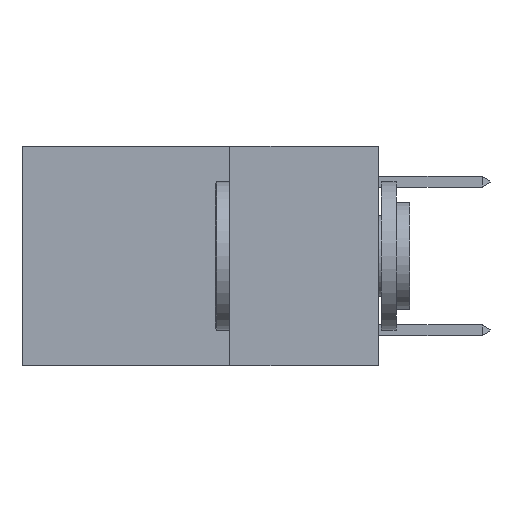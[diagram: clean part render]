
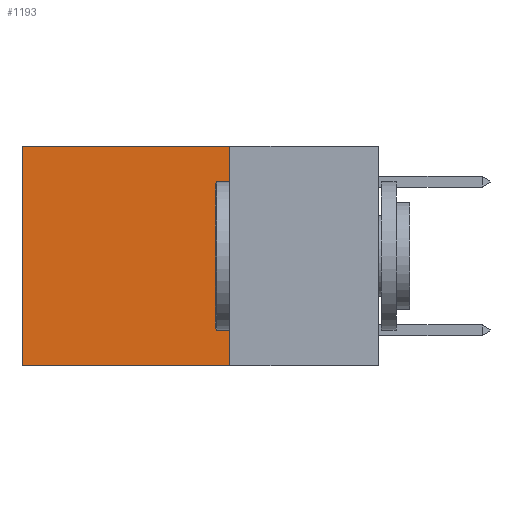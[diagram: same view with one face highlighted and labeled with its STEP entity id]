
A CAD part, left-side view. The second image highlights one B-rep face of the part: STEP entity #1193.
In plain terms, the highlighted planar face has unit normal (-1, 0, 0).
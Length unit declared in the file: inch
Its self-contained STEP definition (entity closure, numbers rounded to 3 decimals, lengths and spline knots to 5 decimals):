
#996 = ORIENTED_EDGE ( 'NONE', *, *, #20381, .F. ) ;
#1029 = LINE ( 'NONE', #21350, #8404 ) ;
#1193 = ADVANCED_FACE ( 'NONE', ( #12612 ), #3220, .F. ) ;
#1572 = CARTESIAN_POINT ( 'NONE',  ( 0.2625, 0.6, 0. ) ) ;
#2079 = DIRECTION ( 'NONE',  ( 0., 1., 0. ) ) ;
#3168 = EDGE_CURVE ( 'NONE', #18322, #13015, #1029, .T. ) ;
#3220 = PLANE ( 'NONE',  #7513 ) ;
#3239 = DIRECTION ( 'NONE',  ( 0., 0., -1. ) ) ;
#3312 = CARTESIAN_POINT ( 'NONE',  ( 0.2625, 0.25, 0. ) ) ;
#4882 = VERTEX_POINT ( 'NONE', #9072 ) ;
#4938 = DIRECTION ( 'NONE',  ( 0., 0., -1. ) ) ;
#7513 = AXIS2_PLACEMENT_3D ( 'NONE', #18361, #14005, #21629 ) ;
#8404 = VECTOR ( 'NONE', #16106, 39.37008 ) ;
#8825 = EDGE_CURVE ( 'NONE', #13015, #11141, #14647, .T. ) ;
#9072 = CARTESIAN_POINT ( 'NONE',  ( 0.2625, 0.25, -0.37 ) ) ;
#9476 = LINE ( 'NONE', #16934, #18950 ) ;
#9788 = EDGE_CURVE ( 'NONE', #18322, #4882, #12326, .T. ) ;
#10072 = CARTESIAN_POINT ( 'NONE',  ( 0.2625, 0.6, 0. ) ) ;
#11141 = VERTEX_POINT ( 'NONE', #22239 ) ;
#11530 = ORIENTED_EDGE ( 'NONE', *, *, #8825, .T. ) ;
#12019 = VECTOR ( 'NONE', #3239, 39.37008 ) ;
#12326 = LINE ( 'NONE', #3312, #16847 ) ;
#12612 = FACE_OUTER_BOUND ( 'NONE', #20590, .T. ) ;
#13015 = VERTEX_POINT ( 'NONE', #10072 ) ;
#14005 = DIRECTION ( 'NONE',  ( 1., 0., 0. ) ) ;
#14647 = LINE ( 'NONE', #1572, #12019 ) ;
#14754 = ORIENTED_EDGE ( 'NONE', *, *, #3168, .T. ) ;
#15773 = ORIENTED_EDGE ( 'NONE', *, *, #9788, .F. ) ;
#16106 = DIRECTION ( 'NONE',  ( 0., 1., 0. ) ) ;
#16847 = VECTOR ( 'NONE', #4938, 39.37008 ) ;
#16934 = CARTESIAN_POINT ( 'NONE',  ( 0.2625, 0.25, -0.37 ) ) ;
#18199 = CARTESIAN_POINT ( 'NONE',  ( 0.2625, 0.25, 0. ) ) ;
#18322 = VERTEX_POINT ( 'NONE', #18199 ) ;
#18361 = CARTESIAN_POINT ( 'NONE',  ( 0.2625, 0.25, 0. ) ) ;
#18950 = VECTOR ( 'NONE', #2079, 39.37008 ) ;
#20381 = EDGE_CURVE ( 'NONE', #4882, #11141, #9476, .T. ) ;
#20590 = EDGE_LOOP ( 'NONE', ( #11530, #996, #15773, #14754 ) ) ;
#21350 = CARTESIAN_POINT ( 'NONE',  ( 0.2625, 0.25, 0. ) ) ;
#21629 = DIRECTION ( 'NONE',  ( 0., 0., -1. ) ) ;
#22239 = CARTESIAN_POINT ( 'NONE',  ( 0.2625, 0.6, -0.37 ) ) ;
